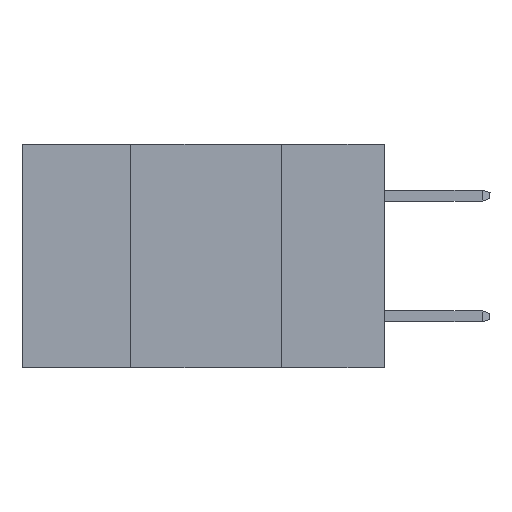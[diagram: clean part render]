
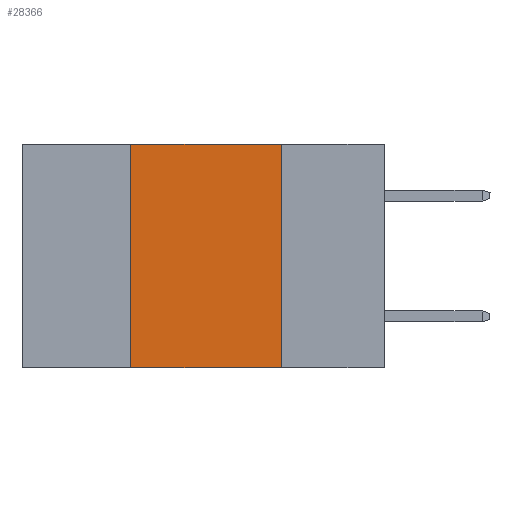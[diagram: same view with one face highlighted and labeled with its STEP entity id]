
A CAD part, left-side view. The second image highlights one B-rep face of the part: STEP entity #28366.
In plain terms, the highlighted planar face has unit normal (-1, 0, 0).
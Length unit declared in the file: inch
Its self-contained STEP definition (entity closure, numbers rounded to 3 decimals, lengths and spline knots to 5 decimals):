
#1027 = CARTESIAN_POINT ( 'NONE',  ( 0., 0.42, -0.37 ) ) ;
#1280 = DIRECTION ( 'NONE',  ( 0., 0., -1. ) ) ;
#1392 = LINE ( 'NONE', #22955, #18189 ) ;
#1553 = LINE ( 'NONE', #17076, #20560 ) ;
#3159 = AXIS2_PLACEMENT_3D ( 'NONE', #3763, #6188, #1280 ) ;
#3763 = CARTESIAN_POINT ( 'NONE',  ( 0., 0.6, 0. ) ) ;
#5125 = VECTOR ( 'NONE', #25647, 39.37008 ) ;
#5333 = EDGE_CURVE ( 'NONE', #29890, #17025, #1392, .T. ) ;
#5902 = LINE ( 'NONE', #20804, #5125 ) ;
#6188 = DIRECTION ( 'NONE',  ( 1., 0., 0. ) ) ;
#8600 = LINE ( 'NONE', #26631, #18633 ) ;
#9246 = EDGE_CURVE ( 'NONE', #17025, #15064, #5902, .T. ) ;
#15064 = VERTEX_POINT ( 'NONE', #26958 ) ;
#15401 = ORIENTED_EDGE ( 'NONE', *, *, #22100, .F. ) ;
#15427 = EDGE_CURVE ( 'NONE', #29890, #26265, #8600, .T. ) ;
#17025 = VERTEX_POINT ( 'NONE', #18838 ) ;
#17076 = CARTESIAN_POINT ( 'NONE',  ( 0., 0.17, 0. ) ) ;
#18189 = VECTOR ( 'NONE', #30077, 39.37008 ) ;
#18633 = VECTOR ( 'NONE', #19625, 39.37008 ) ;
#18757 = CARTESIAN_POINT ( 'NONE',  ( 0., 0.17, -0.37 ) ) ;
#18838 = CARTESIAN_POINT ( 'NONE',  ( 0., 0.42, 0. ) ) ;
#19625 = DIRECTION ( 'NONE',  ( 0., -1., 0. ) ) ;
#20560 = VECTOR ( 'NONE', #21531, 39.37008 ) ;
#20804 = CARTESIAN_POINT ( 'NONE',  ( 0., 0.6, 0. ) ) ;
#21531 = DIRECTION ( 'NONE',  ( 0., 0., -1. ) ) ;
#22100 = EDGE_CURVE ( 'NONE', #15064, #26265, #1553, .T. ) ;
#22955 = CARTESIAN_POINT ( 'NONE',  ( 0., 0.42, 0. ) ) ;
#25647 = DIRECTION ( 'NONE',  ( 0., -1., 0. ) ) ;
#26016 = EDGE_LOOP ( 'NONE', ( #15401, #30455, #27076, #30851 ) ) ;
#26265 = VERTEX_POINT ( 'NONE', #18757 ) ;
#26631 = CARTESIAN_POINT ( 'NONE',  ( 0., 0.6, -0.37 ) ) ;
#26958 = CARTESIAN_POINT ( 'NONE',  ( 0., 0.17, 0. ) ) ;
#27076 = ORIENTED_EDGE ( 'NONE', *, *, #5333, .F. ) ;
#28144 = FACE_OUTER_BOUND ( 'NONE', #26016, .T. ) ;
#28366 = ADVANCED_FACE ( 'NONE', ( #28144 ), #29794, .F. ) ;
#29794 = PLANE ( 'NONE',  #3159 ) ;
#29890 = VERTEX_POINT ( 'NONE', #1027 ) ;
#30077 = DIRECTION ( 'NONE',  ( 0., 0., 1. ) ) ;
#30455 = ORIENTED_EDGE ( 'NONE', *, *, #9246, .F. ) ;
#30851 = ORIENTED_EDGE ( 'NONE', *, *, #15427, .T. ) ;
